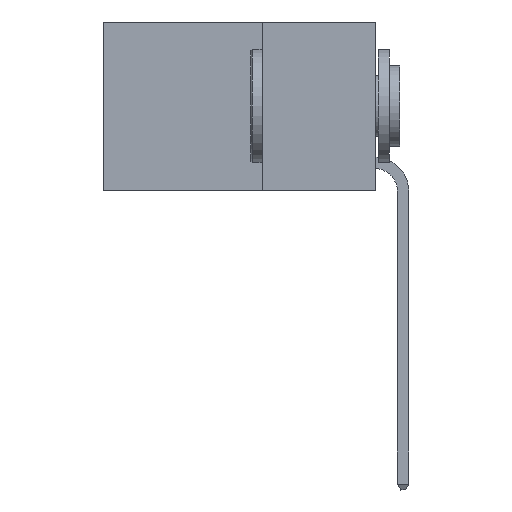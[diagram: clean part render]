
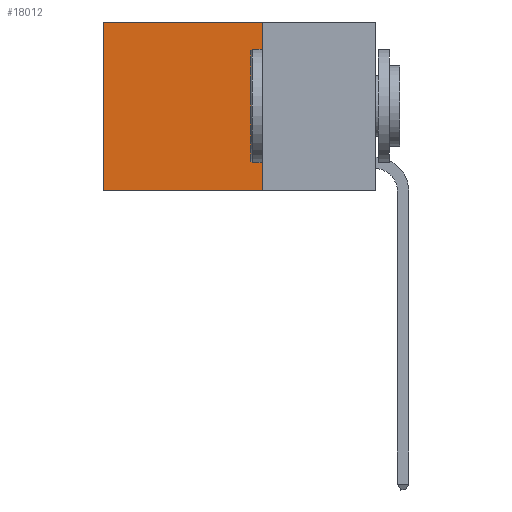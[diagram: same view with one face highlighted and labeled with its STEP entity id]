
A CAD part, left-side view. The second image highlights one B-rep face of the part: STEP entity #18012.
In plain terms, the highlighted planar face has unit normal (-1, 0, 0).
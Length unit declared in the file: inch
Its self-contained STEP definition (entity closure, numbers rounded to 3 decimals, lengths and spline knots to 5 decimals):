
#298 = LINE ( 'NONE', #4738, #5095 ) ;
#660 = ORIENTED_EDGE ( 'NONE', *, *, #4396, .F. ) ;
#1459 = DIRECTION ( 'NONE',  ( 0., 0., -1. ) ) ;
#1520 = VERTEX_POINT ( 'NONE', #20719 ) ;
#2695 = EDGE_CURVE ( 'NONE', #1520, #26536, #298, .T. ) ;
#3751 = LINE ( 'NONE', #5979, #4118 ) ;
#4118 = VECTOR ( 'NONE', #10567, 39.37008 ) ;
#4396 = EDGE_CURVE ( 'NONE', #1520, #25324, #22161, .T. ) ;
#4738 = CARTESIAN_POINT ( 'NONE',  ( 0.2625, 0.25, 0. ) ) ;
#5095 = VECTOR ( 'NONE', #24982, 39.37008 ) ;
#5979 = CARTESIAN_POINT ( 'NONE',  ( 0.2625, 0.6, 0. ) ) ;
#6012 = PLANE ( 'NONE',  #25798 ) ;
#8688 = DIRECTION ( 'NONE',  ( 0., 0., -1. ) ) ;
#8898 = ORIENTED_EDGE ( 'NONE', *, *, #18558, .T. ) ;
#10567 = DIRECTION ( 'NONE',  ( 0., 0., -1. ) ) ;
#12375 = CARTESIAN_POINT ( 'NONE',  ( 0.2625, 0.25, -0.37 ) ) ;
#13185 = ORIENTED_EDGE ( 'NONE', *, *, #16572, .F. ) ;
#13526 = EDGE_LOOP ( 'NONE', ( #8898, #13185, #660, #16409 ) ) ;
#13839 = VERTEX_POINT ( 'NONE', #15034 ) ;
#15034 = CARTESIAN_POINT ( 'NONE',  ( 0.2625, 0.6, -0.37 ) ) ;
#15222 = CARTESIAN_POINT ( 'NONE',  ( 0.2625, 0.25, -0.37 ) ) ;
#16409 = ORIENTED_EDGE ( 'NONE', *, *, #2695, .T. ) ;
#16572 = EDGE_CURVE ( 'NONE', #25324, #13839, #27709, .T. ) ;
#18012 = ADVANCED_FACE ( 'NONE', ( #20192 ), #6012, .F. ) ;
#18370 = VECTOR ( 'NONE', #1459, 39.37008 ) ;
#18558 = EDGE_CURVE ( 'NONE', #26536, #13839, #3751, .T. ) ;
#20192 = FACE_OUTER_BOUND ( 'NONE', #13526, .T. ) ;
#20719 = CARTESIAN_POINT ( 'NONE',  ( 0.2625, 0.25, 0. ) ) ;
#22161 = LINE ( 'NONE', #26590, #18370 ) ;
#22404 = DIRECTION ( 'NONE',  ( 1., 0., 0. ) ) ;
#24400 = VECTOR ( 'NONE', #27987, 39.37008 ) ;
#24471 = CARTESIAN_POINT ( 'NONE',  ( 0.2625, 0.25, 0. ) ) ;
#24982 = DIRECTION ( 'NONE',  ( 0., 1., 0. ) ) ;
#25324 = VERTEX_POINT ( 'NONE', #15222 ) ;
#25798 = AXIS2_PLACEMENT_3D ( 'NONE', #24471, #22404, #8688 ) ;
#26305 = CARTESIAN_POINT ( 'NONE',  ( 0.2625, 0.6, 0. ) ) ;
#26536 = VERTEX_POINT ( 'NONE', #26305 ) ;
#26590 = CARTESIAN_POINT ( 'NONE',  ( 0.2625, 0.25, 0. ) ) ;
#27709 = LINE ( 'NONE', #12375, #24400 ) ;
#27987 = DIRECTION ( 'NONE',  ( 0., 1., 0. ) ) ;
